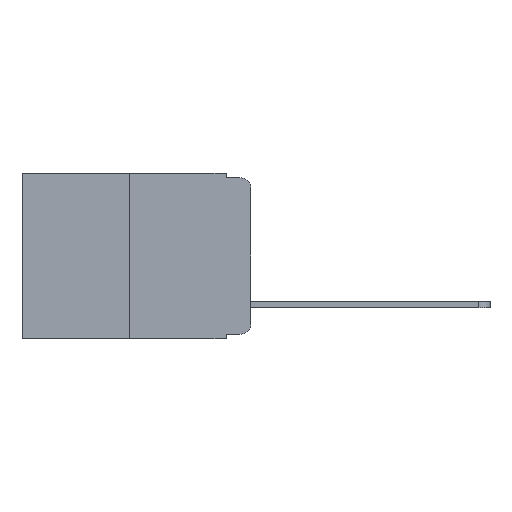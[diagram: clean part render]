
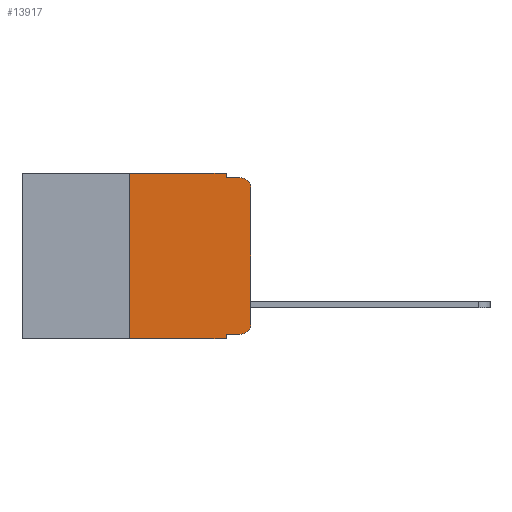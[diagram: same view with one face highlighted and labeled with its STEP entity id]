
A CAD part, left-side view. The second image highlights one B-rep face of the part: STEP entity #13917.
In plain terms, the highlighted planar face has unit normal (-1, 0, 0).
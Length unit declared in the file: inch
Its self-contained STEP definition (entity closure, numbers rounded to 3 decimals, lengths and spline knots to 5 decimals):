
#691 = EDGE_CURVE ( 'NONE', #8612, #7064, #1388, .T. ) ;
#839 = DIRECTION ( 'NONE',  ( -1., 0., 0. ) ) ;
#871 = DIRECTION ( 'NONE',  ( -1., 0., 0. ) ) ;
#1129 = EDGE_CURVE ( 'NONE', #9362, #4548, #16657, .T. ) ;
#1362 = ORIENTED_EDGE ( 'NONE', *, *, #16116, .F. ) ;
#1388 = LINE ( 'NONE', #5877, #16995 ) ;
#1907 = EDGE_CURVE ( 'NONE', #11123, #19612, #10684, .T. ) ;
#2611 = CIRCLE ( 'NONE', #22633, 0.02 ) ;
#3143 = VERTEX_POINT ( 'NONE', #11149 ) ;
#4149 = EDGE_CURVE ( 'NONE', #3143, #7656, #18863, .T. ) ;
#4185 = EDGE_CURVE ( 'NONE', #19612, #14518, #2611, .T. ) ;
#4472 = ORIENTED_EDGE ( 'NONE', *, *, #1907, .T. ) ;
#4548 = VERTEX_POINT ( 'NONE', #20922 ) ;
#5242 = CARTESIAN_POINT ( 'NONE',  ( 0., 0.051, 0. ) ) ;
#5426 = LINE ( 'NONE', #8389, #24758 ) ;
#5827 = EDGE_CURVE ( 'NONE', #8612, #23034, #12355, .T. ) ;
#5877 = CARTESIAN_POINT ( 'NONE',  ( 0., 0.25, 0. ) ) ;
#5883 = ORIENTED_EDGE ( 'NONE', *, *, #691, .F. ) ;
#6258 = VECTOR ( 'NONE', #16872, 39.37008 ) ;
#6278 = CARTESIAN_POINT ( 'NONE',  ( 0., 0.051, -0.343 ) ) ;
#6331 = CARTESIAN_POINT ( 'NONE',  ( 0., 0., -0.313 ) ) ;
#6366 = ORIENTED_EDGE ( 'NONE', *, *, #4149, .T. ) ;
#6849 = DIRECTION ( 'NONE',  ( 0., 0., -1. ) ) ;
#6927 = DIRECTION ( 'NONE',  ( 1., 0., 0. ) ) ;
#7064 = VERTEX_POINT ( 'NONE', #15106 ) ;
#7409 = EDGE_LOOP ( 'NONE', ( #23471, #6366, #1362, #17492, #22492, #5883, #8421, #18274, #4472, #10281 ) ) ;
#7656 = VERTEX_POINT ( 'NONE', #20470 ) ;
#7839 = DIRECTION ( 'NONE',  ( 0., 0., 1. ) ) ;
#8389 = CARTESIAN_POINT ( 'NONE',  ( 0., 0.051, -0.01 ) ) ;
#8421 = ORIENTED_EDGE ( 'NONE', *, *, #5827, .T. ) ;
#8612 = VERTEX_POINT ( 'NONE', #9605 ) ;
#8854 = VECTOR ( 'NONE', #9331, 39.37008 ) ;
#9331 = DIRECTION ( 'NONE',  ( 0., -1., 0. ) ) ;
#9362 = VERTEX_POINT ( 'NONE', #22433 ) ;
#9518 = CARTESIAN_POINT ( 'NONE',  ( 0., 0., 0. ) ) ;
#9605 = CARTESIAN_POINT ( 'NONE',  ( 0., 0.25, -0.343 ) ) ;
#9669 = AXIS2_PLACEMENT_3D ( 'NONE', #18560, #6927, #6849 ) ;
#9706 = DIRECTION ( 'NONE',  ( 0., 0., -1. ) ) ;
#10209 = CARTESIAN_POINT ( 'NONE',  ( 0., 0.473, 0. ) ) ;
#10281 = ORIENTED_EDGE ( 'NONE', *, *, #4185, .T. ) ;
#10342 = CARTESIAN_POINT ( 'NONE',  ( 0., 0.02, -0.333 ) ) ;
#10594 = CARTESIAN_POINT ( 'NONE',  ( 0., 0.02, -0.313 ) ) ;
#10684 = LINE ( 'NONE', #11535, #8854 ) ;
#11123 = VERTEX_POINT ( 'NONE', #24213 ) ;
#11149 = CARTESIAN_POINT ( 'NONE',  ( 0., 0., -0.03 ) ) ;
#11441 = DIRECTION ( 'NONE',  ( 0., -1., 0. ) ) ;
#11453 = VECTOR ( 'NONE', #21181, 39.37008 ) ;
#11535 = CARTESIAN_POINT ( 'NONE',  ( 0., 0.051, -0.333 ) ) ;
#11559 = DIRECTION ( 'NONE',  ( 0., 0., 1. ) ) ;
#12355 = LINE ( 'NONE', #24683, #6258 ) ;
#12462 = LINE ( 'NONE', #15590, #14591 ) ;
#12608 = CARTESIAN_POINT ( 'NONE',  ( 0., 0.02, -0.03 ) ) ;
#13917 = ADVANCED_FACE ( 'NONE', ( #15064 ), #18648, .F. ) ;
#14518 = VERTEX_POINT ( 'NONE', #6331 ) ;
#14567 = DIRECTION ( 'NONE',  ( 0., 0., -1. ) ) ;
#14591 = VECTOR ( 'NONE', #9706, 39.37008 ) ;
#15064 = FACE_OUTER_BOUND ( 'NONE', #7409, .T. ) ;
#15071 = VECTOR ( 'NONE', #11441, 39.37008 ) ;
#15106 = CARTESIAN_POINT ( 'NONE',  ( 0., 0.25, 0. ) ) ;
#15590 = CARTESIAN_POINT ( 'NONE',  ( 0., 0.051, 0. ) ) ;
#16116 = EDGE_CURVE ( 'NONE', #4548, #7656, #5426, .T. ) ;
#16657 = LINE ( 'NONE', #5242, #11453 ) ;
#16872 = DIRECTION ( 'NONE',  ( 0., -1., 0. ) ) ;
#16995 = VECTOR ( 'NONE', #7839, 39.37008 ) ;
#17492 = ORIENTED_EDGE ( 'NONE', *, *, #1129, .F. ) ;
#17747 = VECTOR ( 'NONE', #11559, 39.37008 ) ;
#18150 = LINE ( 'NONE', #10209, #15071 ) ;
#18274 = ORIENTED_EDGE ( 'NONE', *, *, #25096, .F. ) ;
#18494 = DIRECTION ( 'NONE',  ( 0., 0., -1. ) ) ;
#18560 = CARTESIAN_POINT ( 'NONE',  ( 0., 0.473, 0. ) ) ;
#18648 = PLANE ( 'NONE',  #9669 ) ;
#18863 = CIRCLE ( 'NONE', #22484, 0.02 ) ;
#19612 = VERTEX_POINT ( 'NONE', #10342 ) ;
#20470 = CARTESIAN_POINT ( 'NONE',  ( 0., 0.02, -0.01 ) ) ;
#20512 = LINE ( 'NONE', #9518, #17747 ) ;
#20922 = CARTESIAN_POINT ( 'NONE',  ( 0., 0.051, -0.01 ) ) ;
#21181 = DIRECTION ( 'NONE',  ( 0., 0., -1. ) ) ;
#21480 = EDGE_CURVE ( 'NONE', #7064, #9362, #18150, .T. ) ;
#22433 = CARTESIAN_POINT ( 'NONE',  ( 0., 0.051, 0. ) ) ;
#22484 = AXIS2_PLACEMENT_3D ( 'NONE', #12608, #871, #14567 ) ;
#22492 = ORIENTED_EDGE ( 'NONE', *, *, #21480, .F. ) ;
#22630 = EDGE_CURVE ( 'NONE', #14518, #3143, #20512, .T. ) ;
#22633 = AXIS2_PLACEMENT_3D ( 'NONE', #10594, #839, #18494 ) ;
#23034 = VERTEX_POINT ( 'NONE', #6278 ) ;
#23471 = ORIENTED_EDGE ( 'NONE', *, *, #22630, .T. ) ;
#23916 = DIRECTION ( 'NONE',  ( 0., -1., 0. ) ) ;
#24213 = CARTESIAN_POINT ( 'NONE',  ( 0., 0.051, -0.333 ) ) ;
#24683 = CARTESIAN_POINT ( 'NONE',  ( 0., 0.473, -0.343 ) ) ;
#24758 = VECTOR ( 'NONE', #23916, 39.37008 ) ;
#25096 = EDGE_CURVE ( 'NONE', #11123, #23034, #12462, .T. ) ;
